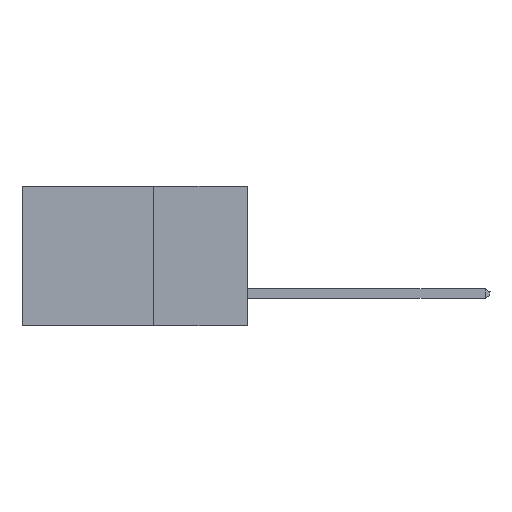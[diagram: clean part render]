
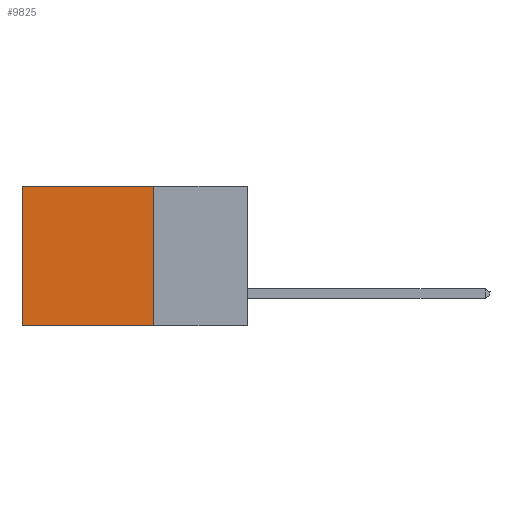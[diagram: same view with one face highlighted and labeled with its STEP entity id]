
A CAD part, left-side view. The second image highlights one B-rep face of the part: STEP entity #9825.
In plain terms, the highlighted planar face has unit normal (-1, 0, 0).
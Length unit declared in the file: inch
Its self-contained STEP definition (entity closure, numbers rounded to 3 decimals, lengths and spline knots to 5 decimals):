
#152 = DIRECTION ( 'NONE',  ( 0., 0., -1. ) ) ;
#756 = DIRECTION ( 'NONE',  ( 0., 1., 0. ) ) ;
#1767 = CARTESIAN_POINT ( 'NONE',  ( 0.2615, 0.6, -0.37 ) ) ;
#2016 = VERTEX_POINT ( 'NONE', #6844 ) ;
#2744 = CARTESIAN_POINT ( 'NONE',  ( 0.2615, 0.25, -0.37 ) ) ;
#4080 = VECTOR ( 'NONE', #11709, 39.37008 ) ;
#4334 = EDGE_CURVE ( 'NONE', #12126, #17797, #4419, .T. ) ;
#4419 = LINE ( 'NONE', #7271, #4080 ) ;
#4747 = ORIENTED_EDGE ( 'NONE', *, *, #12326, .F. ) ;
#5889 = EDGE_CURVE ( 'NONE', #12126, #6953, #17494, .T. ) ;
#6155 = LINE ( 'NONE', #11934, #17261 ) ;
#6489 = EDGE_CURVE ( 'NONE', #17797, #2016, #14720, .T. ) ;
#6660 = AXIS2_PLACEMENT_3D ( 'NONE', #17288, #8949, #152 ) ;
#6844 = CARTESIAN_POINT ( 'NONE',  ( 0.2615, 0.6, -0.37 ) ) ;
#6953 = VERTEX_POINT ( 'NONE', #2744 ) ;
#7271 = CARTESIAN_POINT ( 'NONE',  ( 0.2615, 0.25, 0. ) ) ;
#7541 = DIRECTION ( 'NONE',  ( 0., 0., -1. ) ) ;
#8949 = DIRECTION ( 'NONE',  ( 1., 0., 0. ) ) ;
#9825 = ADVANCED_FACE ( 'NONE', ( #17565 ), #10465, .F. ) ;
#10140 = CARTESIAN_POINT ( 'NONE',  ( 0.2615, 0.25, 0. ) ) ;
#10298 = DIRECTION ( 'NONE',  ( 0., 0., -1. ) ) ;
#10465 = PLANE ( 'NONE',  #6660 ) ;
#11416 = VECTOR ( 'NONE', #7541, 39.37008 ) ;
#11709 = DIRECTION ( 'NONE',  ( 0., 1., 0. ) ) ;
#11838 = CARTESIAN_POINT ( 'NONE',  ( 0.2615, 0.6, 0. ) ) ;
#11934 = CARTESIAN_POINT ( 'NONE',  ( 0.2615, 0.25, -0.37 ) ) ;
#12126 = VERTEX_POINT ( 'NONE', #10140 ) ;
#12326 = EDGE_CURVE ( 'NONE', #6953, #2016, #6155, .T. ) ;
#13006 = ORIENTED_EDGE ( 'NONE', *, *, #4334, .T. ) ;
#14720 = LINE ( 'NONE', #1767, #11416 ) ;
#15240 = ORIENTED_EDGE ( 'NONE', *, *, #6489, .T. ) ;
#15708 = CARTESIAN_POINT ( 'NONE',  ( 0.2615, 0.25, -0.37 ) ) ;
#16047 = ORIENTED_EDGE ( 'NONE', *, *, #5889, .F. ) ;
#17261 = VECTOR ( 'NONE', #756, 39.37008 ) ;
#17288 = CARTESIAN_POINT ( 'NONE',  ( 0.2615, 0.25, -0.37 ) ) ;
#17421 = EDGE_LOOP ( 'NONE', ( #15240, #4747, #16047, #13006 ) ) ;
#17494 = LINE ( 'NONE', #15708, #18351 ) ;
#17565 = FACE_OUTER_BOUND ( 'NONE', #17421, .T. ) ;
#17797 = VERTEX_POINT ( 'NONE', #11838 ) ;
#18351 = VECTOR ( 'NONE', #10298, 39.37008 ) ;
